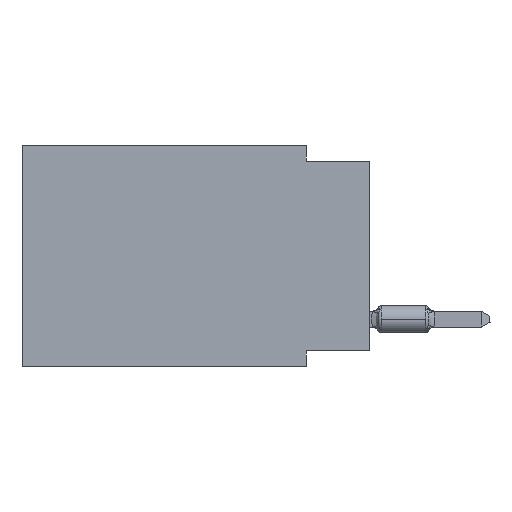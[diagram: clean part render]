
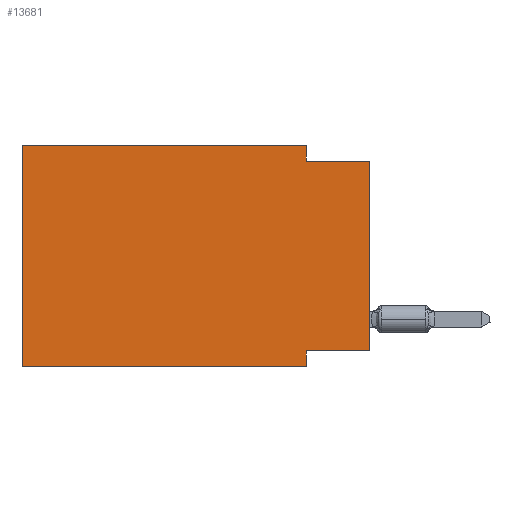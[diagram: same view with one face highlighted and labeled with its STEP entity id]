
A CAD part, left-side view. The second image highlights one B-rep face of the part: STEP entity #13681.
In plain terms, the highlighted planar face has unit normal (-1, 0, 0).
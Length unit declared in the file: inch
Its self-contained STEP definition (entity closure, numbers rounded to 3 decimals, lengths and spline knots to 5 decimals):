
#139 = LINE ( 'NONE', #24783, #46110 ) ;
#490 = EDGE_CURVE ( 'NONE', #59048, #34857, #28691, .T. ) ;
#1087 = LINE ( 'NONE', #59139, #4130 ) ;
#1589 = EDGE_CURVE ( 'NONE', #43529, #14933, #1087, .T. ) ;
#2845 = CARTESIAN_POINT ( 'NONE',  ( 0., 0.1, -0.35 ) ) ;
#3912 = VECTOR ( 'NONE', #29905, 39.37008 ) ;
#4130 = VECTOR ( 'NONE', #11363, 39.37008 ) ;
#4231 = CARTESIAN_POINT ( 'NONE',  ( 0., 0.55, -0.35 ) ) ;
#5148 = DIRECTION ( 'NONE',  ( 0., -1., 0. ) ) ;
#5835 = EDGE_CURVE ( 'NONE', #59048, #32981, #44871, .T. ) ;
#7360 = DIRECTION ( 'NONE',  ( 0., 0., -1. ) ) ;
#8018 = CARTESIAN_POINT ( 'NONE',  ( 0., 0.1, 0. ) ) ;
#9030 = CARTESIAN_POINT ( 'NONE',  ( 0., 0.55, -0.35 ) ) ;
#11037 = CARTESIAN_POINT ( 'NONE',  ( 0., 0.55, 0. ) ) ;
#11159 = CARTESIAN_POINT ( 'NONE',  ( 0., 0., 0. ) ) ;
#11363 = DIRECTION ( 'NONE',  ( 0., 0., 1. ) ) ;
#13681 = ADVANCED_FACE ( 'NONE', ( #47605 ), #53509, .F. ) ;
#14933 = VERTEX_POINT ( 'NONE', #59117 ) ;
#15914 = CARTESIAN_POINT ( 'NONE',  ( 0., 0.1, -0.325 ) ) ;
#16149 = ORIENTED_EDGE ( 'NONE', *, *, #490, .F. ) ;
#17766 = EDGE_CURVE ( 'NONE', #34512, #32981, #139, .T. ) ;
#18702 = EDGE_LOOP ( 'NONE', ( #26095, #27532, #22785, #60701, #48469, #52793, #53458, #16149 ) ) ;
#20102 = LINE ( 'NONE', #11037, #27736 ) ;
#20408 = DIRECTION ( 'NONE',  ( 0., -1., 0. ) ) ;
#22116 = VECTOR ( 'NONE', #7360, 39.37008 ) ;
#22487 = LINE ( 'NONE', #2845, #29586 ) ;
#22785 = ORIENTED_EDGE ( 'NONE', *, *, #25297, .F. ) ;
#24480 = CARTESIAN_POINT ( 'NONE',  ( 0., 0.55, 0. ) ) ;
#24783 = CARTESIAN_POINT ( 'NONE',  ( 0., 0., -0.025 ) ) ;
#24968 = CARTESIAN_POINT ( 'NONE',  ( 0., 0.1, -0.35 ) ) ;
#25297 = EDGE_CURVE ( 'NONE', #59339, #34512, #31075, .T. ) ;
#26095 = ORIENTED_EDGE ( 'NONE', *, *, #5835, .T. ) ;
#27532 = ORIENTED_EDGE ( 'NONE', *, *, #17766, .F. ) ;
#27736 = VECTOR ( 'NONE', #20408, 39.37008 ) ;
#27738 = CARTESIAN_POINT ( 'NONE',  ( 0., 0., -0.325 ) ) ;
#28522 = EDGE_CURVE ( 'NONE', #43529, #31965, #60865, .T. ) ;
#28691 = LINE ( 'NONE', #37435, #33254 ) ;
#29586 = VECTOR ( 'NONE', #61442, 39.37008 ) ;
#29905 = DIRECTION ( 'NONE',  ( 0., 0., 1. ) ) ;
#31075 = LINE ( 'NONE', #53588, #22116 ) ;
#31296 = CARTESIAN_POINT ( 'NONE',  ( 0., 0.1, -0.025 ) ) ;
#31965 = VERTEX_POINT ( 'NONE', #24968 ) ;
#32981 = VERTEX_POINT ( 'NONE', #40747 ) ;
#33254 = VECTOR ( 'NONE', #56476, 39.37008 ) ;
#34512 = VERTEX_POINT ( 'NONE', #31296 ) ;
#34857 = VERTEX_POINT ( 'NONE', #15914 ) ;
#37435 = CARTESIAN_POINT ( 'NONE',  ( 0., 0., -0.325 ) ) ;
#40747 = CARTESIAN_POINT ( 'NONE',  ( 0., 0., -0.025 ) ) ;
#43067 = DIRECTION ( 'NONE',  ( 0., -1., 0. ) ) ;
#43529 = VERTEX_POINT ( 'NONE', #4231 ) ;
#44316 = EDGE_CURVE ( 'NONE', #34857, #31965, #22487, .T. ) ;
#44871 = LINE ( 'NONE', #11159, #3912 ) ;
#46110 = VECTOR ( 'NONE', #5148, 39.37008 ) ;
#47605 = FACE_OUTER_BOUND ( 'NONE', #18702, .T. ) ;
#47907 = DIRECTION ( 'NONE',  ( 1., 0., 0. ) ) ;
#47994 = EDGE_CURVE ( 'NONE', #14933, #59339, #20102, .T. ) ;
#48469 = ORIENTED_EDGE ( 'NONE', *, *, #1589, .F. ) ;
#49885 = AXIS2_PLACEMENT_3D ( 'NONE', #24480, #47907, #52890 ) ;
#52793 = ORIENTED_EDGE ( 'NONE', *, *, #28522, .T. ) ;
#52890 = DIRECTION ( 'NONE',  ( 0., 0., -1. ) ) ;
#53458 = ORIENTED_EDGE ( 'NONE', *, *, #44316, .F. ) ;
#53509 = PLANE ( 'NONE',  #49885 ) ;
#53588 = CARTESIAN_POINT ( 'NONE',  ( 0., 0.1, 0. ) ) ;
#56178 = VECTOR ( 'NONE', #43067, 39.37008 ) ;
#56476 = DIRECTION ( 'NONE',  ( 0., 1., 0. ) ) ;
#59048 = VERTEX_POINT ( 'NONE', #27738 ) ;
#59117 = CARTESIAN_POINT ( 'NONE',  ( 0., 0.55, 0. ) ) ;
#59139 = CARTESIAN_POINT ( 'NONE',  ( 0., 0.55, 0. ) ) ;
#59339 = VERTEX_POINT ( 'NONE', #8018 ) ;
#60701 = ORIENTED_EDGE ( 'NONE', *, *, #47994, .F. ) ;
#60865 = LINE ( 'NONE', #9030, #56178 ) ;
#61442 = DIRECTION ( 'NONE',  ( 0., 0., -1. ) ) ;
